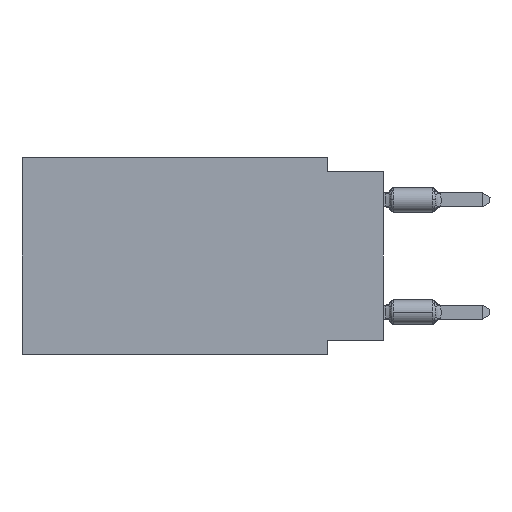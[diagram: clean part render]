
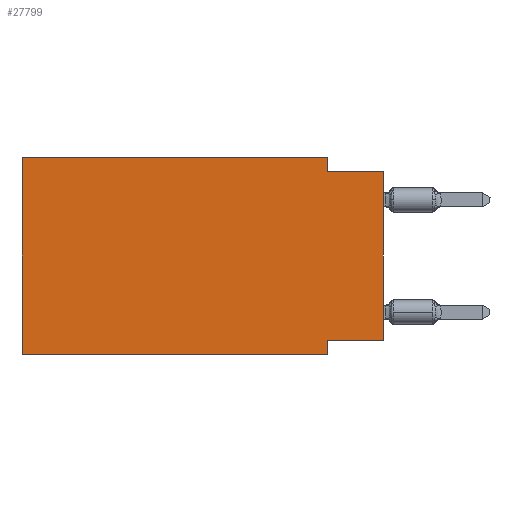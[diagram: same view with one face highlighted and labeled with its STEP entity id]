
A CAD part, left-side view. The second image highlights one B-rep face of the part: STEP entity #27799.
In plain terms, the highlighted planar face has unit normal (-1, 0, 0).
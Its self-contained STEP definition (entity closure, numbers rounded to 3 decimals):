
#420 = VECTOR ( 'NONE', #14627, 1000. ) ;
#442 = VERTEX_POINT ( 'NONE', #9057 ) ;
#547 = VERTEX_POINT ( 'NONE', #18284 ) ;
#981 = VERTEX_POINT ( 'NONE', #31164 ) ;
#1507 = LINE ( 'NONE', #8987, #24626 ) ;
#2431 = EDGE_CURVE ( 'NONE', #547, #7893, #28066, .T. ) ;
#2682 = VECTOR ( 'NONE', #9697, 1000. ) ;
#4210 = EDGE_CURVE ( 'NONE', #981, #9551, #23925, .T. ) ;
#5826 = CARTESIAN_POINT ( 'NONE',  ( 0., 2.54, -8.89 ) ) ;
#6842 = CARTESIAN_POINT ( 'NONE',  ( 0., 0., -8.255 ) ) ;
#7024 = CARTESIAN_POINT ( 'NONE',  ( 0., 16.383, 0. ) ) ;
#7083 = CARTESIAN_POINT ( 'NONE',  ( 0., 16.383, 0. ) ) ;
#7221 = DIRECTION ( 'NONE',  ( 0., 0., -1. ) ) ;
#7390 = ORIENTED_EDGE ( 'NONE', *, *, #17848, .T. ) ;
#7893 = VERTEX_POINT ( 'NONE', #27447 ) ;
#8292 = CARTESIAN_POINT ( 'NONE',  ( 0., 16.383, 0. ) ) ;
#8472 = VECTOR ( 'NONE', #22524, 1000. ) ;
#8598 = LINE ( 'NONE', #8951, #420 ) ;
#8599 = LINE ( 'NONE', #16419, #30427 ) ;
#8951 = CARTESIAN_POINT ( 'NONE',  ( 0., 0., 0. ) ) ;
#8987 = CARTESIAN_POINT ( 'NONE',  ( 0., 16.383, -8.89 ) ) ;
#9057 = CARTESIAN_POINT ( 'NONE',  ( 0., 2.54, 0. ) ) ;
#9062 = EDGE_CURVE ( 'NONE', #16092, #18975, #23432, .T. ) ;
#9324 = AXIS2_PLACEMENT_3D ( 'NONE', #11820, #30828, #25328 ) ;
#9551 = VERTEX_POINT ( 'NONE', #5826 ) ;
#9697 = DIRECTION ( 'NONE',  ( 0., -1., 0. ) ) ;
#9930 = DIRECTION ( 'NONE',  ( 0., 0., 1. ) ) ;
#9981 = EDGE_CURVE ( 'NONE', #31863, #7893, #8598, .T. ) ;
#10051 = ORIENTED_EDGE ( 'NONE', *, *, #9981, .T. ) ;
#10408 = ORIENTED_EDGE ( 'NONE', *, *, #19287, .F. ) ;
#11128 = ORIENTED_EDGE ( 'NONE', *, *, #9062, .F. ) ;
#11820 = CARTESIAN_POINT ( 'NONE',  ( 0., 16.383, 0. ) ) ;
#12672 = EDGE_LOOP ( 'NONE', ( #10051, #24787, #10408, #34697, #11128, #7390, #33696, #22187 ) ) ;
#13794 = VECTOR ( 'NONE', #31086, 1000. ) ;
#14627 = DIRECTION ( 'NONE',  ( 0., 0., 1. ) ) ;
#15748 = CARTESIAN_POINT ( 'NONE',  ( 0., 2.54, -8.89 ) ) ;
#16092 = VERTEX_POINT ( 'NONE', #18787 ) ;
#16419 = CARTESIAN_POINT ( 'NONE',  ( 0., 2.54, 0. ) ) ;
#17325 = PLANE ( 'NONE',  #9324 ) ;
#17689 = DIRECTION ( 'NONE',  ( 0., -1., 0. ) ) ;
#17848 = EDGE_CURVE ( 'NONE', #16092, #9551, #1507, .T. ) ;
#18284 = CARTESIAN_POINT ( 'NONE',  ( 0., 2.54, -0.635 ) ) ;
#18624 = VECTOR ( 'NONE', #9930, 1000. ) ;
#18787 = CARTESIAN_POINT ( 'NONE',  ( 0., 16.383, -8.89 ) ) ;
#18975 = VERTEX_POINT ( 'NONE', #8292 ) ;
#19287 = EDGE_CURVE ( 'NONE', #442, #547, #8599, .T. ) ;
#20215 = EDGE_CURVE ( 'NONE', #18975, #442, #34057, .T. ) ;
#22168 = LINE ( 'NONE', #30702, #8472 ) ;
#22187 = ORIENTED_EDGE ( 'NONE', *, *, #23704, .F. ) ;
#22524 = DIRECTION ( 'NONE',  ( 0., 1., 0. ) ) ;
#23432 = LINE ( 'NONE', #7083, #18624 ) ;
#23704 = EDGE_CURVE ( 'NONE', #31863, #981, #22168, .T. ) ;
#23883 = VECTOR ( 'NONE', #7221, 1000. ) ;
#23925 = LINE ( 'NONE', #15748, #23883 ) ;
#24626 = VECTOR ( 'NONE', #17689, 1000. ) ;
#24764 = DIRECTION ( 'NONE',  ( 0., 0., -1. ) ) ;
#24787 = ORIENTED_EDGE ( 'NONE', *, *, #2431, .F. ) ;
#25328 = DIRECTION ( 'NONE',  ( 0., 0., -1. ) ) ;
#27447 = CARTESIAN_POINT ( 'NONE',  ( 0., 0., -0.635 ) ) ;
#27799 = ADVANCED_FACE ( 'NONE', ( #31193 ), #17325, .F. ) ;
#28066 = LINE ( 'NONE', #30902, #13794 ) ;
#30427 = VECTOR ( 'NONE', #24764, 1000. ) ;
#30702 = CARTESIAN_POINT ( 'NONE',  ( 0., 0., -8.255 ) ) ;
#30828 = DIRECTION ( 'NONE',  ( 1., 0., 0. ) ) ;
#30902 = CARTESIAN_POINT ( 'NONE',  ( 0., 0., -0.635 ) ) ;
#31086 = DIRECTION ( 'NONE',  ( 0., -1., 0. ) ) ;
#31164 = CARTESIAN_POINT ( 'NONE',  ( 0., 2.54, -8.255 ) ) ;
#31193 = FACE_OUTER_BOUND ( 'NONE', #12672, .T. ) ;
#31863 = VERTEX_POINT ( 'NONE', #6842 ) ;
#33696 = ORIENTED_EDGE ( 'NONE', *, *, #4210, .F. ) ;
#34057 = LINE ( 'NONE', #7024, #2682 ) ;
#34697 = ORIENTED_EDGE ( 'NONE', *, *, #20215, .F. ) ;
